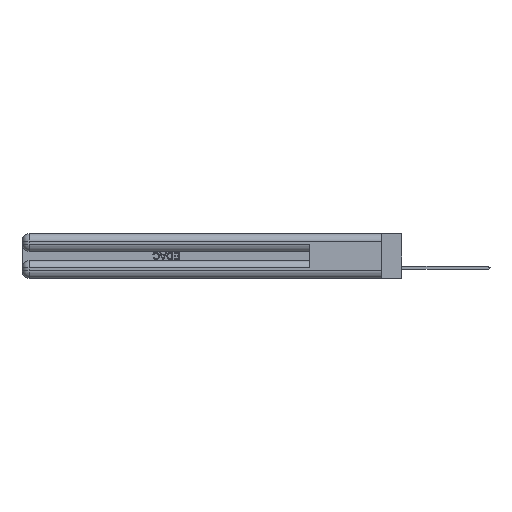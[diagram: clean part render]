
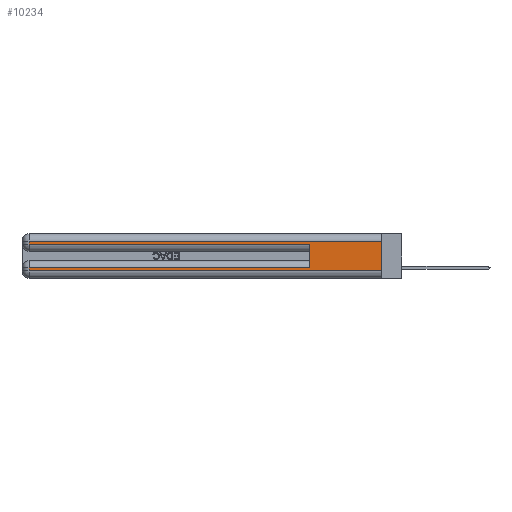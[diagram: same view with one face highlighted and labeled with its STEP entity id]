
A CAD part, left-side view. The second image highlights one B-rep face of the part: STEP entity #10234.
In plain terms, the highlighted planar face has unit normal (-1, 0, 0).
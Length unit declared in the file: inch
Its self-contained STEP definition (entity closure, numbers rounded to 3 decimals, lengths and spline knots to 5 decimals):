
#48 = DIRECTION ( 'NONE',  ( 0., 1., 0. ) ) ;
#1031 = VECTOR ( 'NONE', #25158, 39.37008 ) ;
#1072 = EDGE_CURVE ( 'NONE', #37812, #37116, #14776, .T. ) ;
#1840 = LINE ( 'NONE', #31134, #29558 ) ;
#2277 = VECTOR ( 'NONE', #5361, 39.37008 ) ;
#2311 = DIRECTION ( 'NONE',  ( 0., 0., 1. ) ) ;
#2736 = LINE ( 'NONE', #20486, #18372 ) ;
#2909 = CARTESIAN_POINT ( 'NONE',  ( 0., 2.94, 0.06 ) ) ;
#3379 = VERTEX_POINT ( 'NONE', #12455 ) ;
#4410 = EDGE_CURVE ( 'NONE', #24982, #35470, #1840, .T. ) ;
#4863 = FACE_OUTER_BOUND ( 'NONE', #13585, .T. ) ;
#5028 = CARTESIAN_POINT ( 'NONE',  ( 0., 0., 0.31 ) ) ;
#5361 = DIRECTION ( 'NONE',  ( 0., 0., -1. ) ) ;
#6094 = LINE ( 'NONE', #5028, #41034 ) ;
#6339 = DIRECTION ( 'NONE',  ( 0., 0., -1. ) ) ;
#9025 = VECTOR ( 'NONE', #2311, 39.37008 ) ;
#9832 = VERTEX_POINT ( 'NONE', #15514 ) ;
#10234 = ADVANCED_FACE ( 'NONE', ( #4863 ), #30473, .F. ) ;
#10580 = LINE ( 'NONE', #31541, #1031 ) ;
#10888 = DIRECTION ( 'NONE',  ( 0., 1., 0. ) ) ;
#11043 = EDGE_CURVE ( 'NONE', #37812, #9832, #28301, .T. ) ;
#11323 = LINE ( 'NONE', #24582, #2277 ) ;
#12455 = CARTESIAN_POINT ( 'NONE',  ( 0., 2.94, 0.285 ) ) ;
#13485 = EDGE_CURVE ( 'NONE', #37116, #25595, #11323, .T. ) ;
#13585 = EDGE_LOOP ( 'NONE', ( #26394, #20902, #25257, #37618, #20575, #29400, #31025, #41161 ) ) ;
#13588 = EDGE_CURVE ( 'NONE', #32412, #3379, #30553, .T. ) ;
#14035 = DIRECTION ( 'NONE',  ( 1., 0., 0. ) ) ;
#14776 = LINE ( 'NONE', #41896, #38580 ) ;
#15514 = CARTESIAN_POINT ( 'NONE',  ( 0., 0.6, 0.285 ) ) ;
#16362 = EDGE_CURVE ( 'NONE', #24982, #32412, #6094, .T. ) ;
#17234 = CARTESIAN_POINT ( 'NONE',  ( 0., 2.94, 0.37 ) ) ;
#18372 = VECTOR ( 'NONE', #30107, 39.37008 ) ;
#20486 = CARTESIAN_POINT ( 'NONE',  ( 0., 0., 0.06 ) ) ;
#20575 = ORIENTED_EDGE ( 'NONE', *, *, #11043, .F. ) ;
#20902 = ORIENTED_EDGE ( 'NONE', *, *, #16362, .T. ) ;
#22089 = EDGE_CURVE ( 'NONE', #25595, #35470, #2736, .T. ) ;
#23363 = CARTESIAN_POINT ( 'NONE',  ( 0., 0.6, 0.085 ) ) ;
#24182 = CARTESIAN_POINT ( 'NONE',  ( 0., 2.94, 0.085 ) ) ;
#24582 = CARTESIAN_POINT ( 'NONE',  ( 0., 2.94, 0.37 ) ) ;
#24982 = VERTEX_POINT ( 'NONE', #28280 ) ;
#25158 = DIRECTION ( 'NONE',  ( 0., -1., 0. ) ) ;
#25257 = ORIENTED_EDGE ( 'NONE', *, *, #13588, .T. ) ;
#25595 = VERTEX_POINT ( 'NONE', #2909 ) ;
#26394 = ORIENTED_EDGE ( 'NONE', *, *, #4410, .F. ) ;
#26647 = DIRECTION ( 'NONE',  ( 0., 0., -1. ) ) ;
#28001 = CARTESIAN_POINT ( 'NONE',  ( 0., 2.94, 0.31 ) ) ;
#28280 = CARTESIAN_POINT ( 'NONE',  ( 0., 0., 0.31 ) ) ;
#28301 = LINE ( 'NONE', #34100, #9025 ) ;
#29400 = ORIENTED_EDGE ( 'NONE', *, *, #1072, .T. ) ;
#29558 = VECTOR ( 'NONE', #6339, 39.37008 ) ;
#30107 = DIRECTION ( 'NONE',  ( 0., -1., 0. ) ) ;
#30473 = PLANE ( 'NONE',  #40262 ) ;
#30553 = LINE ( 'NONE', #17234, #36083 ) ;
#31025 = ORIENTED_EDGE ( 'NONE', *, *, #13485, .T. ) ;
#31134 = CARTESIAN_POINT ( 'NONE',  ( 0., 0., 0.37 ) ) ;
#31541 = CARTESIAN_POINT ( 'NONE',  ( 0., 0., 0.285 ) ) ;
#32412 = VERTEX_POINT ( 'NONE', #28001 ) ;
#32677 = EDGE_CURVE ( 'NONE', #3379, #9832, #10580, .T. ) ;
#33124 = CARTESIAN_POINT ( 'NONE',  ( 0., 0., 0.37 ) ) ;
#34100 = CARTESIAN_POINT ( 'NONE',  ( 0., 0.6, 0.145 ) ) ;
#35470 = VERTEX_POINT ( 'NONE', #37676 ) ;
#36083 = VECTOR ( 'NONE', #39891, 39.37008 ) ;
#37116 = VERTEX_POINT ( 'NONE', #24182 ) ;
#37618 = ORIENTED_EDGE ( 'NONE', *, *, #32677, .T. ) ;
#37676 = CARTESIAN_POINT ( 'NONE',  ( 0., 0., 0.06 ) ) ;
#37812 = VERTEX_POINT ( 'NONE', #23363 ) ;
#38580 = VECTOR ( 'NONE', #48, 39.37008 ) ;
#39891 = DIRECTION ( 'NONE',  ( 0., 0., -1. ) ) ;
#40262 = AXIS2_PLACEMENT_3D ( 'NONE', #33124, #14035, #26647 ) ;
#41034 = VECTOR ( 'NONE', #10888, 39.37008 ) ;
#41161 = ORIENTED_EDGE ( 'NONE', *, *, #22089, .T. ) ;
#41896 = CARTESIAN_POINT ( 'NONE',  ( 0., 0., 0.085 ) ) ;
